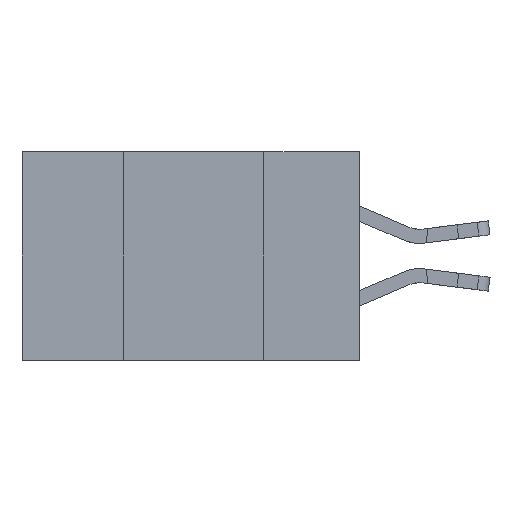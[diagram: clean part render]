
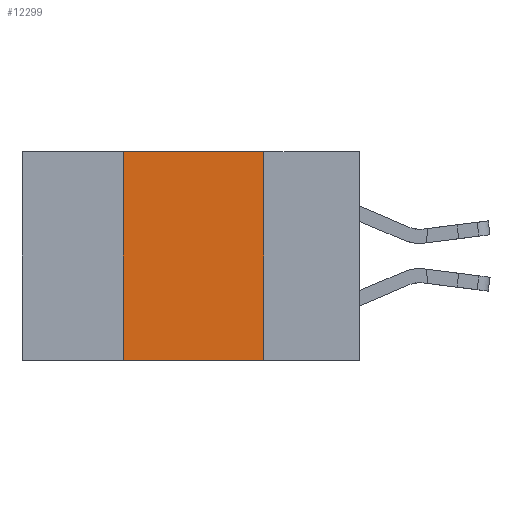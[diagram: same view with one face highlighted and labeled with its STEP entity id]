
A CAD part, left-side view. The second image highlights one B-rep face of the part: STEP entity #12299.
In plain terms, the highlighted planar face has unit normal (-1, 0, 0).
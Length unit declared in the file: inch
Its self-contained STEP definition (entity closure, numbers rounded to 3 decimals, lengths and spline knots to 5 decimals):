
#327 = VERTEX_POINT ( 'NONE', #24248 ) ;
#1139 = LINE ( 'NONE', #4558, #10919 ) ;
#2569 = EDGE_CURVE ( 'NONE', #15803, #21090, #1139, .T. ) ;
#4103 = EDGE_CURVE ( 'NONE', #16478, #21090, #10164, .T. ) ;
#4558 = CARTESIAN_POINT ( 'NONE',  ( 0., 0.6, -0.37 ) ) ;
#4754 = DIRECTION ( 'NONE',  ( 0., -1., 0. ) ) ;
#6156 = CARTESIAN_POINT ( 'NONE',  ( 0., 0.42, 0. ) ) ;
#6605 = ORIENTED_EDGE ( 'NONE', *, *, #4103, .F. ) ;
#6628 = DIRECTION ( 'NONE',  ( 0., 0., -1. ) ) ;
#6839 = CARTESIAN_POINT ( 'NONE',  ( 0., 0.17, 0. ) ) ;
#8755 = DIRECTION ( 'NONE',  ( 0., -1., 0. ) ) ;
#8876 = VECTOR ( 'NONE', #6628, 39.37008 ) ;
#9577 = EDGE_CURVE ( 'NONE', #327, #16478, #10317, .T. ) ;
#10164 = LINE ( 'NONE', #15018, #8876 ) ;
#10168 = CARTESIAN_POINT ( 'NONE',  ( 0., 0.6, 0. ) ) ;
#10317 = LINE ( 'NONE', #25286, #26254 ) ;
#10682 = ORIENTED_EDGE ( 'NONE', *, *, #2569, .T. ) ;
#10919 = VECTOR ( 'NONE', #4754, 39.37008 ) ;
#11493 = EDGE_LOOP ( 'NONE', ( #6605, #26247, #12064, #10682 ) ) ;
#12064 = ORIENTED_EDGE ( 'NONE', *, *, #26344, .F. ) ;
#12299 = ADVANCED_FACE ( 'NONE', ( #17352 ), #18383, .F. ) ;
#14381 = VECTOR ( 'NONE', #18826, 39.37008 ) ;
#15018 = CARTESIAN_POINT ( 'NONE',  ( 0., 0.17, 0. ) ) ;
#15803 = VERTEX_POINT ( 'NONE', #26045 ) ;
#16394 = DIRECTION ( 'NONE',  ( 1., 0., 0. ) ) ;
#16478 = VERTEX_POINT ( 'NONE', #6839 ) ;
#17352 = FACE_OUTER_BOUND ( 'NONE', #11493, .T. ) ;
#18383 = PLANE ( 'NONE',  #23307 ) ;
#18826 = DIRECTION ( 'NONE',  ( 0., 0., 1. ) ) ;
#21090 = VERTEX_POINT ( 'NONE', #24218 ) ;
#21517 = LINE ( 'NONE', #6156, #14381 ) ;
#23307 = AXIS2_PLACEMENT_3D ( 'NONE', #10168, #16394, #24791 ) ;
#24218 = CARTESIAN_POINT ( 'NONE',  ( 0., 0.17, -0.37 ) ) ;
#24248 = CARTESIAN_POINT ( 'NONE',  ( 0., 0.42, 0. ) ) ;
#24791 = DIRECTION ( 'NONE',  ( 0., 0., -1. ) ) ;
#25286 = CARTESIAN_POINT ( 'NONE',  ( 0., 0.6, 0. ) ) ;
#26045 = CARTESIAN_POINT ( 'NONE',  ( 0., 0.42, -0.37 ) ) ;
#26247 = ORIENTED_EDGE ( 'NONE', *, *, #9577, .F. ) ;
#26254 = VECTOR ( 'NONE', #8755, 39.37008 ) ;
#26344 = EDGE_CURVE ( 'NONE', #15803, #327, #21517, .T. ) ;
